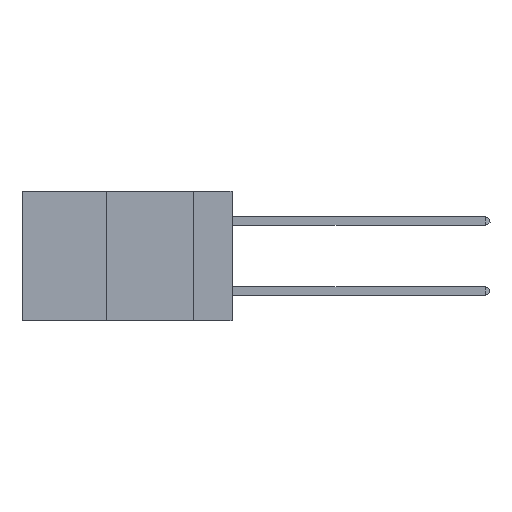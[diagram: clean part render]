
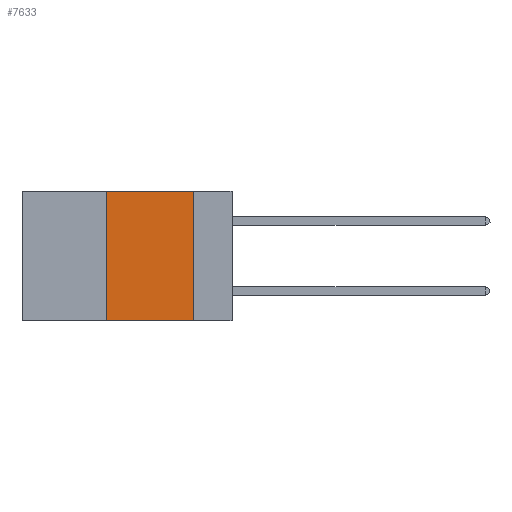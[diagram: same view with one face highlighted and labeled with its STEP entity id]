
A CAD part, left-side view. The second image highlights one B-rep face of the part: STEP entity #7633.
In plain terms, the highlighted planar face has unit normal (-1, 0, 0).
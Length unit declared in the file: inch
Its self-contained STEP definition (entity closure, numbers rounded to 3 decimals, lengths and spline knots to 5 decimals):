
#41 = CARTESIAN_POINT ( 'NONE',  ( 0., 0.36, -0.37 ) ) ;
#62 = EDGE_CURVE ( 'NONE', #10926, #12367, #807, .T. ) ;
#120 = DIRECTION ( 'NONE',  ( 0., 0., -1. ) ) ;
#348 = CARTESIAN_POINT ( 'NONE',  ( 0., 0.36, 0. ) ) ;
#387 = ORIENTED_EDGE ( 'NONE', *, *, #10802, .T. ) ;
#807 = LINE ( 'NONE', #10044, #4233 ) ;
#1516 = EDGE_CURVE ( 'NONE', #6217, #10926, #9899, .T. ) ;
#1619 = CARTESIAN_POINT ( 'NONE',  ( 0., 0.6, -0.37 ) ) ;
#1858 = ORIENTED_EDGE ( 'NONE', *, *, #62, .F. ) ;
#2744 = CARTESIAN_POINT ( 'NONE',  ( 0., 0.11, 0. ) ) ;
#4233 = VECTOR ( 'NONE', #4509, 39.37008 ) ;
#4509 = DIRECTION ( 'NONE',  ( 0., 0., -1. ) ) ;
#4787 = ORIENTED_EDGE ( 'NONE', *, *, #4904, .F. ) ;
#4904 = EDGE_CURVE ( 'NONE', #11116, #6217, #10775, .T. ) ;
#5353 = AXIS2_PLACEMENT_3D ( 'NONE', #6064, #9908, #120 ) ;
#5690 = VECTOR ( 'NONE', #8128, 39.37008 ) ;
#6064 = CARTESIAN_POINT ( 'NONE',  ( 0., 0.6, 0. ) ) ;
#6217 = VERTEX_POINT ( 'NONE', #6866 ) ;
#6341 = VECTOR ( 'NONE', #11484, 39.37008 ) ;
#6466 = ORIENTED_EDGE ( 'NONE', *, *, #1516, .F. ) ;
#6822 = VECTOR ( 'NONE', #9823, 39.37008 ) ;
#6866 = CARTESIAN_POINT ( 'NONE',  ( 0., 0.36, 0. ) ) ;
#7633 = ADVANCED_FACE ( 'NONE', ( #9770 ), #10847, .F. ) ;
#8128 = DIRECTION ( 'NONE',  ( 0., 0., 1. ) ) ;
#8973 = CARTESIAN_POINT ( 'NONE',  ( 0., 0.6, 0. ) ) ;
#9770 = FACE_OUTER_BOUND ( 'NONE', #9832, .T. ) ;
#9823 = DIRECTION ( 'NONE',  ( 0., -1., 0. ) ) ;
#9832 = EDGE_LOOP ( 'NONE', ( #1858, #6466, #4787, #387 ) ) ;
#9899 = LINE ( 'NONE', #8973, #6822 ) ;
#9908 = DIRECTION ( 'NONE',  ( 1., 0., 0. ) ) ;
#10044 = CARTESIAN_POINT ( 'NONE',  ( 0., 0.11, 0. ) ) ;
#10626 = CARTESIAN_POINT ( 'NONE',  ( 0., 0.11, -0.37 ) ) ;
#10775 = LINE ( 'NONE', #348, #5690 ) ;
#10802 = EDGE_CURVE ( 'NONE', #11116, #12367, #11713, .T. ) ;
#10847 = PLANE ( 'NONE',  #5353 ) ;
#10926 = VERTEX_POINT ( 'NONE', #2744 ) ;
#11116 = VERTEX_POINT ( 'NONE', #41 ) ;
#11484 = DIRECTION ( 'NONE',  ( 0., -1., 0. ) ) ;
#11713 = LINE ( 'NONE', #1619, #6341 ) ;
#12367 = VERTEX_POINT ( 'NONE', #10626 ) ;
